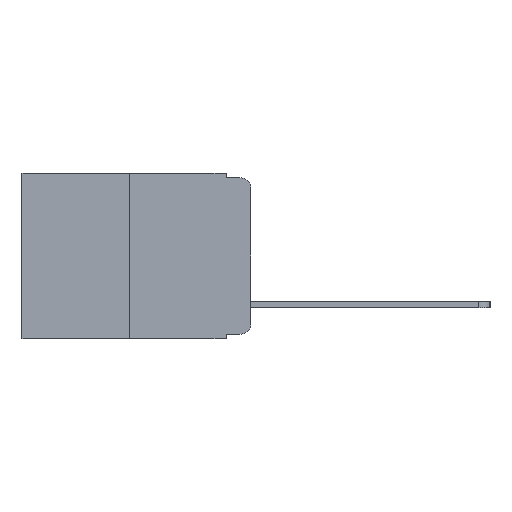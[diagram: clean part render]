
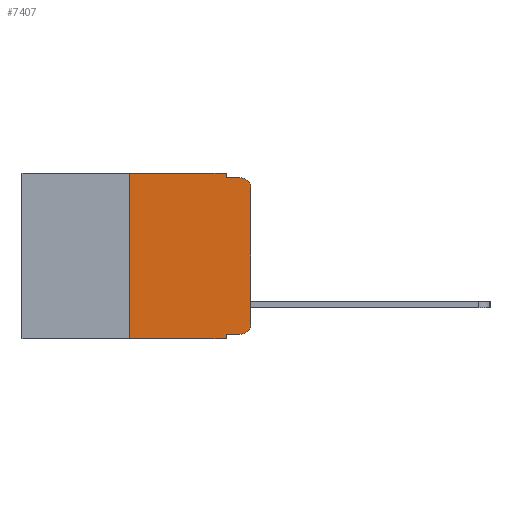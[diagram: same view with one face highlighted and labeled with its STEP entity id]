
A CAD part, left-side view. The second image highlights one B-rep face of the part: STEP entity #7407.
In plain terms, the highlighted planar face has unit normal (-1, 0, 0).
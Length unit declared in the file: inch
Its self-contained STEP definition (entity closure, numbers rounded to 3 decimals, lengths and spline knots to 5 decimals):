
#193 = ORIENTED_EDGE ( 'NONE', *, *, #5975, .T. ) ;
#267 = CARTESIAN_POINT ( 'NONE',  ( 0., 0.051, 0. ) ) ;
#371 = DIRECTION ( 'NONE',  ( 0., 0., -1. ) ) ;
#500 = CARTESIAN_POINT ( 'NONE',  ( 0., 0., 0. ) ) ;
#598 = CIRCLE ( 'NONE', #11199, 0.02 ) ;
#1334 = ORIENTED_EDGE ( 'NONE', *, *, #10381, .T. ) ;
#1371 = ORIENTED_EDGE ( 'NONE', *, *, #10741, .T. ) ;
#1429 = DIRECTION ( 'NONE',  ( 0., 0., -1. ) ) ;
#1544 = LINE ( 'NONE', #5206, #10696 ) ;
#1633 = ORIENTED_EDGE ( 'NONE', *, *, #10948, .F. ) ;
#1773 = ORIENTED_EDGE ( 'NONE', *, *, #11219, .F. ) ;
#1841 = DIRECTION ( 'NONE',  ( 0., -1., 0. ) ) ;
#1955 = CARTESIAN_POINT ( 'NONE',  ( 0., 0.02, -0.333 ) ) ;
#2101 = CARTESIAN_POINT ( 'NONE',  ( 0., 0.473, -0.343 ) ) ;
#2109 = ORIENTED_EDGE ( 'NONE', *, *, #7425, .F. ) ;
#2210 = VERTEX_POINT ( 'NONE', #1955 ) ;
#2226 = ORIENTED_EDGE ( 'NONE', *, *, #11491, .F. ) ;
#2623 = VECTOR ( 'NONE', #10616, 39.37008 ) ;
#2692 = DIRECTION ( 'NONE',  ( 0., 0., 1. ) ) ;
#2711 = ORIENTED_EDGE ( 'NONE', *, *, #7856, .T. ) ;
#2722 = VECTOR ( 'NONE', #1429, 39.37008 ) ;
#2909 = CARTESIAN_POINT ( 'NONE',  ( 0., 0.25, 0. ) ) ;
#2945 = CARTESIAN_POINT ( 'NONE',  ( 0., 0.051, -0.343 ) ) ;
#3132 = ORIENTED_EDGE ( 'NONE', *, *, #7012, .F. ) ;
#3394 = ORIENTED_EDGE ( 'NONE', *, *, #10006, .T. ) ;
#3846 = DIRECTION ( 'NONE',  ( 0., 0., -1. ) ) ;
#3864 = VECTOR ( 'NONE', #9780, 39.37008 ) ;
#3899 = VERTEX_POINT ( 'NONE', #2945 ) ;
#4010 = AXIS2_PLACEMENT_3D ( 'NONE', #5116, #5344, #5375 ) ;
#4062 = LINE ( 'NONE', #9092, #6133 ) ;
#4071 = VERTEX_POINT ( 'NONE', #6706 ) ;
#4110 = VERTEX_POINT ( 'NONE', #5486 ) ;
#4135 = LINE ( 'NONE', #2101, #10404 ) ;
#4167 = VERTEX_POINT ( 'NONE', #8254 ) ;
#4181 = LINE ( 'NONE', #2909, #10981 ) ;
#4782 = CIRCLE ( 'NONE', #9480, 0.02 ) ;
#5116 = CARTESIAN_POINT ( 'NONE',  ( 0., 0.473, 0. ) ) ;
#5202 = DIRECTION ( 'NONE',  ( 0., 0., -1. ) ) ;
#5206 = CARTESIAN_POINT ( 'NONE',  ( 0., 0.051, 0. ) ) ;
#5344 = DIRECTION ( 'NONE',  ( 1., 0., 0. ) ) ;
#5364 = EDGE_LOOP ( 'NONE', ( #1334, #1371, #1633, #1773, #2109, #2226, #2711, #3132, #3394, #193 ) ) ;
#5375 = DIRECTION ( 'NONE',  ( 0., 0., -1. ) ) ;
#5486 = CARTESIAN_POINT ( 'NONE',  ( 0., 0.02, -0.01 ) ) ;
#5733 = LINE ( 'NONE', #6118, #2722 ) ;
#5805 = VERTEX_POINT ( 'NONE', #267 ) ;
#5975 = EDGE_CURVE ( 'NONE', #2210, #6059, #598, .T. ) ;
#6059 = VERTEX_POINT ( 'NONE', #9079 ) ;
#6118 = CARTESIAN_POINT ( 'NONE',  ( 0., 0.051, 0. ) ) ;
#6133 = VECTOR ( 'NONE', #9921, 39.37008 ) ;
#6193 = DIRECTION ( 'NONE',  ( -1., 0., 0. ) ) ;
#6680 = CARTESIAN_POINT ( 'NONE',  ( 0., 0.051, -0.01 ) ) ;
#6706 = CARTESIAN_POINT ( 'NONE',  ( 0., 0.25, -0.343 ) ) ;
#6782 = VERTEX_POINT ( 'NONE', #9584 ) ;
#7012 = EDGE_CURVE ( 'NONE', #8991, #3899, #1544, .T. ) ;
#7077 = CARTESIAN_POINT ( 'NONE',  ( 0., 0.02, -0.313 ) ) ;
#7094 = DIRECTION ( 'NONE',  ( -1., 0., 0. ) ) ;
#7341 = LINE ( 'NONE', #10612, #2623 ) ;
#7407 = ADVANCED_FACE ( 'NONE', ( #8740 ), #9479, .F. ) ;
#7425 = EDGE_CURVE ( 'NONE', #6782, #5805, #10682, .T. ) ;
#7593 = VECTOR ( 'NONE', #2692, 39.37008 ) ;
#7856 = EDGE_CURVE ( 'NONE', #4071, #3899, #4135, .T. ) ;
#8146 = DIRECTION ( 'NONE',  ( 0., 0., 1. ) ) ;
#8254 = CARTESIAN_POINT ( 'NONE',  ( 0., 0., -0.03 ) ) ;
#8490 = VERTEX_POINT ( 'NONE', #6680 ) ;
#8740 = FACE_OUTER_BOUND ( 'NONE', #5364, .T. ) ;
#8991 = VERTEX_POINT ( 'NONE', #11597 ) ;
#9079 = CARTESIAN_POINT ( 'NONE',  ( 0., 0., -0.313 ) ) ;
#9092 = CARTESIAN_POINT ( 'NONE',  ( 0., 0.051, -0.01 ) ) ;
#9479 = PLANE ( 'NONE',  #4010 ) ;
#9480 = AXIS2_PLACEMENT_3D ( 'NONE', #11229, #6193, #371 ) ;
#9584 = CARTESIAN_POINT ( 'NONE',  ( 0., 0.25, 0. ) ) ;
#9597 = LINE ( 'NONE', #500, #7593 ) ;
#9780 = DIRECTION ( 'NONE',  ( 0., -1., 0. ) ) ;
#9921 = DIRECTION ( 'NONE',  ( 0., -1., 0. ) ) ;
#9953 = CARTESIAN_POINT ( 'NONE',  ( 0., 0.473, 0. ) ) ;
#10006 = EDGE_CURVE ( 'NONE', #8991, #2210, #7341, .T. ) ;
#10381 = EDGE_CURVE ( 'NONE', #6059, #4167, #9597, .T. ) ;
#10404 = VECTOR ( 'NONE', #1841, 39.37008 ) ;
#10612 = CARTESIAN_POINT ( 'NONE',  ( 0., 0.051, -0.333 ) ) ;
#10616 = DIRECTION ( 'NONE',  ( 0., -1., 0. ) ) ;
#10682 = LINE ( 'NONE', #9953, #3864 ) ;
#10696 = VECTOR ( 'NONE', #5202, 39.37008 ) ;
#10741 = EDGE_CURVE ( 'NONE', #4167, #4110, #4782, .T. ) ;
#10948 = EDGE_CURVE ( 'NONE', #8490, #4110, #4062, .T. ) ;
#10981 = VECTOR ( 'NONE', #8146, 39.37008 ) ;
#11199 = AXIS2_PLACEMENT_3D ( 'NONE', #7077, #7094, #3846 ) ;
#11219 = EDGE_CURVE ( 'NONE', #5805, #8490, #5733, .T. ) ;
#11229 = CARTESIAN_POINT ( 'NONE',  ( 0., 0.02, -0.03 ) ) ;
#11491 = EDGE_CURVE ( 'NONE', #4071, #6782, #4181, .T. ) ;
#11597 = CARTESIAN_POINT ( 'NONE',  ( 0., 0.051, -0.333 ) ) ;
